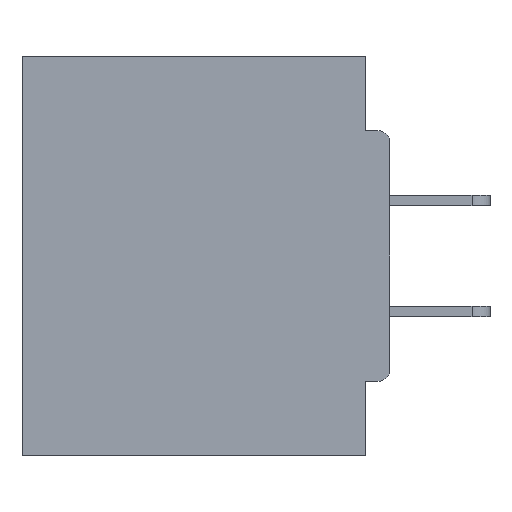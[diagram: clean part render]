
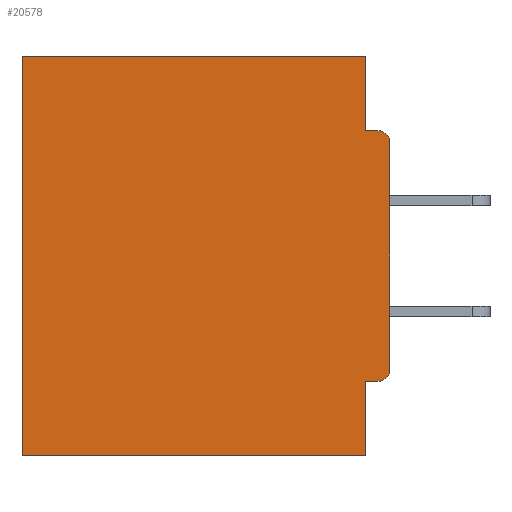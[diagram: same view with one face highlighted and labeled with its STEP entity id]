
A CAD part, left-side view. The second image highlights one B-rep face of the part: STEP entity #20578.
In plain terms, the highlighted planar face has unit normal (-1, 0, 0).
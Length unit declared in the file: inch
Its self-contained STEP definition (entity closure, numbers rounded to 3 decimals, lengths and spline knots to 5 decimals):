
#259 = CARTESIAN_POINT ( 'NONE',  ( 0.298, 0.46, 0. ) ) ;
#353 = AXIS2_PLACEMENT_3D ( 'NONE', #24568, #9608, #17329 ) ;
#390 = EDGE_CURVE ( 'NONE', #3904, #17680, #15472, .T. ) ;
#1213 = DIRECTION ( 'NONE',  ( 0., 1., 0. ) ) ;
#1998 = CARTESIAN_POINT ( 'NONE',  ( 0.298, 0., -0.0935 ) ) ;
#3299 = ORIENTED_EDGE ( 'NONE', *, *, #28016, .F. ) ;
#3540 = LINE ( 'NONE', #25933, #31055 ) ;
#3904 = VERTEX_POINT ( 'NONE', #14667 ) ;
#3972 = EDGE_CURVE ( 'NONE', #3904, #23570, #12853, .T. ) ;
#4913 = ORIENTED_EDGE ( 'NONE', *, *, #10979, .F. ) ;
#5595 = VECTOR ( 'NONE', #32248, 39.37008 ) ;
#5796 = VECTOR ( 'NONE', #18833, 39.37008 ) ;
#6239 = CARTESIAN_POINT ( 'NONE',  ( 0.298, 0.015, -0.0935 ) ) ;
#7679 = LINE ( 'NONE', #259, #32444 ) ;
#7805 = EDGE_CURVE ( 'NONE', #24206, #17680, #8720, .T. ) ;
#8051 = VECTOR ( 'NONE', #14059, 39.37008 ) ;
#8417 = CARTESIAN_POINT ( 'NONE',  ( 0.298, 0., 0. ) ) ;
#8720 = LINE ( 'NONE', #1998, #5595 ) ;
#9497 = ORIENTED_EDGE ( 'NONE', *, *, #7805, .F. ) ;
#9608 = DIRECTION ( 'NONE',  ( -1., 0., 0. ) ) ;
#9947 = AXIS2_PLACEMENT_3D ( 'NONE', #24559, #31732, #29530 ) ;
#10010 = DIRECTION ( 'NONE',  ( 0., 0., -1. ) ) ;
#10979 = EDGE_CURVE ( 'NONE', #11319, #28264, #3540, .T. ) ;
#11319 = VERTEX_POINT ( 'NONE', #11497 ) ;
#11467 = DIRECTION ( 'NONE',  ( 0., 0., -1. ) ) ;
#11497 = CARTESIAN_POINT ( 'NONE',  ( 0.298, 0.031, -0.5 ) ) ;
#11554 = VECTOR ( 'NONE', #12768, 39.37008 ) ;
#12012 = FACE_OUTER_BOUND ( 'NONE', #30034, .T. ) ;
#12720 = CARTESIAN_POINT ( 'NONE',  ( 0.298, 0.031, -0.4065 ) ) ;
#12768 = DIRECTION ( 'NONE',  ( 0., 0., -1. ) ) ;
#12853 = LINE ( 'NONE', #26214, #5796 ) ;
#14006 = ORIENTED_EDGE ( 'NONE', *, *, #29765, .F. ) ;
#14059 = DIRECTION ( 'NONE',  ( 0., 1., 0. ) ) ;
#14096 = CARTESIAN_POINT ( 'NONE',  ( 0.298, 0.031, -0.5 ) ) ;
#14210 = VERTEX_POINT ( 'NONE', #18217 ) ;
#14413 = DIRECTION ( 'NONE',  ( 1., 0., 0. ) ) ;
#14667 = CARTESIAN_POINT ( 'NONE',  ( 0.298, 0., -0.1085 ) ) ;
#15074 = CARTESIAN_POINT ( 'NONE',  ( 0.298, 0.031, -0.5 ) ) ;
#15472 = CIRCLE ( 'NONE', #9947, 0.015 ) ;
#15790 = EDGE_CURVE ( 'NONE', #18317, #29978, #23664, .T. ) ;
#17329 = DIRECTION ( 'NONE',  ( 0., 0., -1. ) ) ;
#17680 = VERTEX_POINT ( 'NONE', #6239 ) ;
#18217 = CARTESIAN_POINT ( 'NONE',  ( 0.298, 0.015, -0.4065 ) ) ;
#18246 = ORIENTED_EDGE ( 'NONE', *, *, #29080, .T. ) ;
#18317 = VERTEX_POINT ( 'NONE', #18919 ) ;
#18833 = DIRECTION ( 'NONE',  ( 0., 0., -1. ) ) ;
#18919 = CARTESIAN_POINT ( 'NONE',  ( 0.298, 0.031, 0. ) ) ;
#20578 = ADVANCED_FACE ( 'NONE', ( #12012 ), #22022, .F. ) ;
#20980 = LINE ( 'NONE', #14096, #23347 ) ;
#21401 = CARTESIAN_POINT ( 'NONE',  ( 0.298, 0., -0.3915 ) ) ;
#22022 = PLANE ( 'NONE',  #30469 ) ;
#23347 = VECTOR ( 'NONE', #11467, 39.37008 ) ;
#23570 = VERTEX_POINT ( 'NONE', #21401 ) ;
#23664 = LINE ( 'NONE', #8417, #27235 ) ;
#24206 = VERTEX_POINT ( 'NONE', #27323 ) ;
#24559 = CARTESIAN_POINT ( 'NONE',  ( 0.298, 0.015, -0.1085 ) ) ;
#24568 = CARTESIAN_POINT ( 'NONE',  ( 0.298, 0.015, -0.3915 ) ) ;
#24882 = CARTESIAN_POINT ( 'NONE',  ( 0.298, 0., 0. ) ) ;
#24950 = LINE ( 'NONE', #15074, #11554 ) ;
#25677 = ORIENTED_EDGE ( 'NONE', *, *, #29275, .T. ) ;
#25689 = ORIENTED_EDGE ( 'NONE', *, *, #3972, .F. ) ;
#25933 = CARTESIAN_POINT ( 'NONE',  ( 0.298, 0., -0.5 ) ) ;
#26214 = CARTESIAN_POINT ( 'NONE',  ( 0.298, 0., 0. ) ) ;
#26876 = ORIENTED_EDGE ( 'NONE', *, *, #15790, .T. ) ;
#27106 = DIRECTION ( 'NONE',  ( 0., 0., -1. ) ) ;
#27126 = ORIENTED_EDGE ( 'NONE', *, *, #31548, .F. ) ;
#27226 = VERTEX_POINT ( 'NONE', #12720 ) ;
#27235 = VECTOR ( 'NONE', #1213, 39.37008 ) ;
#27323 = CARTESIAN_POINT ( 'NONE',  ( 0.298, 0.031, -0.0935 ) ) ;
#27433 = CIRCLE ( 'NONE', #353, 0.015 ) ;
#28016 = EDGE_CURVE ( 'NONE', #18317, #24206, #24950, .T. ) ;
#28264 = VERTEX_POINT ( 'NONE', #29625 ) ;
#28937 = CARTESIAN_POINT ( 'NONE',  ( 0.298, 0., -0.4065 ) ) ;
#29080 = EDGE_CURVE ( 'NONE', #29978, #28264, #7679, .T. ) ;
#29275 = EDGE_CURVE ( 'NONE', #14210, #23570, #27433, .T. ) ;
#29530 = DIRECTION ( 'NONE',  ( 0., 0., -1. ) ) ;
#29625 = CARTESIAN_POINT ( 'NONE',  ( 0.298, 0.46, -0.5 ) ) ;
#29765 = EDGE_CURVE ( 'NONE', #14210, #27226, #30922, .T. ) ;
#29978 = VERTEX_POINT ( 'NONE', #30735 ) ;
#30034 = EDGE_LOOP ( 'NONE', ( #30234, #9497, #3299, #26876, #18246, #4913, #27126, #14006, #25677, #25689 ) ) ;
#30234 = ORIENTED_EDGE ( 'NONE', *, *, #390, .T. ) ;
#30469 = AXIS2_PLACEMENT_3D ( 'NONE', #24882, #14413, #27106 ) ;
#30735 = CARTESIAN_POINT ( 'NONE',  ( 0.298, 0.46, 0. ) ) ;
#30781 = DIRECTION ( 'NONE',  ( 0., 1., 0. ) ) ;
#30922 = LINE ( 'NONE', #28937, #8051 ) ;
#31055 = VECTOR ( 'NONE', #30781, 39.37008 ) ;
#31548 = EDGE_CURVE ( 'NONE', #27226, #11319, #20980, .T. ) ;
#31732 = DIRECTION ( 'NONE',  ( -1., 0., 0. ) ) ;
#32248 = DIRECTION ( 'NONE',  ( 0., -1., 0. ) ) ;
#32444 = VECTOR ( 'NONE', #10010, 39.37008 ) ;
